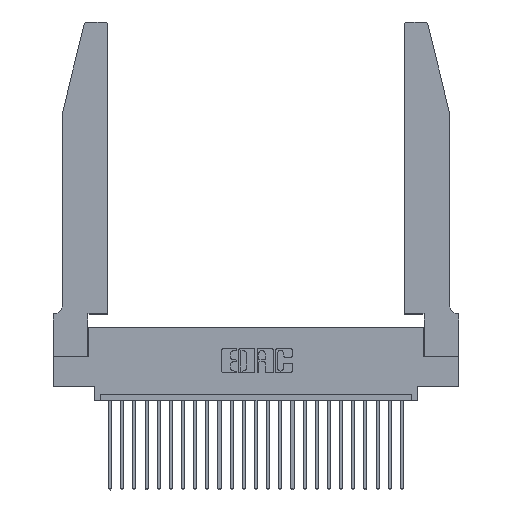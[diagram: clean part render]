
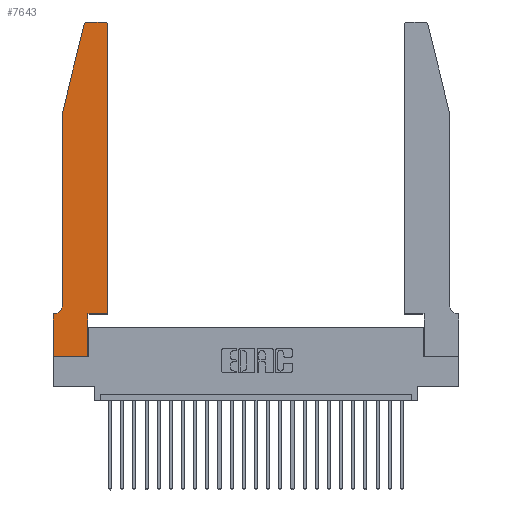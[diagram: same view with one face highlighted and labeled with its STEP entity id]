
A CAD part, top view. The second image highlights one B-rep face of the part: STEP entity #7643.
In plain terms, the highlighted planar face has unit normal (0, 0, 1).
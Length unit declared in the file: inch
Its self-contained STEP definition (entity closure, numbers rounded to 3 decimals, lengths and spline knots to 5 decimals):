
#42 = EDGE_CURVE ( 'NONE', #4178, #14159, #10183, .T. ) ;
#282 = VECTOR ( 'NONE', #21362, 39.37008 ) ;
#537 = DIRECTION ( 'NONE',  ( 1., 0., 0. ) ) ;
#866 = AXIS2_PLACEMENT_3D ( 'NONE', #18104, #2823, #10908 ) ;
#1161 = EDGE_LOOP ( 'NONE', ( #21668, #25241, #9745, #19186, #22105, #18938, #23691, #1825, #6431, #4393, #26007, #18659 ) ) ;
#1350 = CIRCLE ( 'NONE', #866, 0.07 ) ;
#1559 = LINE ( 'NONE', #8080, #11611 ) ;
#1583 = CARTESIAN_POINT ( 'NONE',  ( 0., 0.35, 0.37 ) ) ;
#1825 = ORIENTED_EDGE ( 'NONE', *, *, #9039, .T. ) ;
#1847 = EDGE_CURVE ( 'NONE', #8274, #24404, #5391, .T. ) ;
#2293 = DIRECTION ( 'NONE',  ( 0., 1., 0. ) ) ;
#2823 = DIRECTION ( 'NONE',  ( 0., 0., -1. ) ) ;
#2844 = VECTOR ( 'NONE', #20369, 39.37008 ) ;
#3102 = CARTESIAN_POINT ( 'NONE',  ( 0.0755, 2., 0.37 ) ) ;
#3602 = EDGE_CURVE ( 'NONE', #6146, #17665, #1559, .T. ) ;
#3891 = CARTESIAN_POINT ( 'NONE',  ( 0.2605, 2.75, 0.37 ) ) ;
#4178 = VERTEX_POINT ( 'NONE', #21834 ) ;
#4284 = VERTEX_POINT ( 'NONE', #10160 ) ;
#4393 = ORIENTED_EDGE ( 'NONE', *, *, #17517, .T. ) ;
#4582 = VECTOR ( 'NONE', #25202, 39.37008 ) ;
#4914 = EDGE_CURVE ( 'NONE', #7433, #5770, #16569, .T. ) ;
#5391 = LINE ( 'NONE', #12675, #2844 ) ;
#5650 = DIRECTION ( 'NONE',  ( 0., -1., 0. ) ) ;
#5770 = VERTEX_POINT ( 'NONE', #8282 ) ;
#5902 = CARTESIAN_POINT ( 'NONE',  ( 0.4205, 2.75, 0.37 ) ) ;
#6146 = VERTEX_POINT ( 'NONE', #6194 ) ;
#6194 = CARTESIAN_POINT ( 'NONE',  ( 0., 0.35, 0.37 ) ) ;
#6374 = FACE_OUTER_BOUND ( 'NONE', #1161, .T. ) ;
#6431 = ORIENTED_EDGE ( 'NONE', *, *, #18869, .T. ) ;
#6601 = CARTESIAN_POINT ( 'NONE',  ( 0.2865, 0.35, 0.37 ) ) ;
#6682 = LINE ( 'NONE', #3891, #6994 ) ;
#6994 = VECTOR ( 'NONE', #24303, 39.37008 ) ;
#7001 = EDGE_CURVE ( 'NONE', #5770, #8465, #1350, .T. ) ;
#7410 = CARTESIAN_POINT ( 'NONE',  ( 0.25487, 2.72718, 0.37 ) ) ;
#7433 = VERTEX_POINT ( 'NONE', #19551 ) ;
#7643 = ADVANCED_FACE ( 'NONE', ( #6374 ), #21573, .T. ) ;
#7696 = DIRECTION ( 'NONE',  ( 1., 0., 0. ) ) ;
#8080 = CARTESIAN_POINT ( 'NONE',  ( 0., 0., 0.37 ) ) ;
#8274 = VERTEX_POINT ( 'NONE', #15698 ) ;
#8282 = CARTESIAN_POINT ( 'NONE',  ( 0.0755, 0.42, 0.37 ) ) ;
#8408 = LINE ( 'NONE', #3102, #25663 ) ;
#8465 = VERTEX_POINT ( 'NONE', #17090 ) ;
#9039 = EDGE_CURVE ( 'NONE', #17665, #4284, #26032, .T. ) ;
#9628 = VECTOR ( 'NONE', #2293, 39.37008 ) ;
#9745 = ORIENTED_EDGE ( 'NONE', *, *, #18416, .T. ) ;
#9931 = CARTESIAN_POINT ( 'NONE',  ( 0.0755, 2., 0.37 ) ) ;
#10160 = CARTESIAN_POINT ( 'NONE',  ( 0.2865, 0., 0.37 ) ) ;
#10183 = CIRCLE ( 'NONE', #14211, 0.03 ) ;
#10206 = CIRCLE ( 'NONE', #21078, 0.03 ) ;
#10581 = VERTEX_POINT ( 'NONE', #24111 ) ;
#10833 = LINE ( 'NONE', #19227, #4582 ) ;
#10908 = DIRECTION ( 'NONE',  ( -1., 0., 0. ) ) ;
#11016 = VERTEX_POINT ( 'NONE', #5902 ) ;
#11131 = CARTESIAN_POINT ( 'NONE',  ( 0.4205, 2.72, 0.37 ) ) ;
#11213 = LINE ( 'NONE', #6601, #9628 ) ;
#11611 = VECTOR ( 'NONE', #15700, 39.37008 ) ;
#12675 = CARTESIAN_POINT ( 'NONE',  ( 0.4505, 0.35, 0.37 ) ) ;
#13285 = CARTESIAN_POINT ( 'NONE',  ( 0.4505, 0.35, 0.37 ) ) ;
#13693 = CARTESIAN_POINT ( 'NONE',  ( 0.284, 2.72, 0.37 ) ) ;
#13778 = DIRECTION ( 'NONE',  ( 0., 0., 1. ) ) ;
#14159 = VERTEX_POINT ( 'NONE', #7410 ) ;
#14211 = AXIS2_PLACEMENT_3D ( 'NONE', #13693, #13778, #17656 ) ;
#15086 = DIRECTION ( 'NONE',  ( 0., 0., 1. ) ) ;
#15698 = CARTESIAN_POINT ( 'NONE',  ( 0.4505, 0.35, 0.37 ) ) ;
#15700 = DIRECTION ( 'NONE',  ( 0., -1., 0. ) ) ;
#15930 = EDGE_CURVE ( 'NONE', #11016, #4178, #6682, .T. ) ;
#16569 = LINE ( 'NONE', #9931, #20604 ) ;
#16924 = DIRECTION ( 'NONE',  ( 1., 0., 0. ) ) ;
#17090 = CARTESIAN_POINT ( 'NONE',  ( 0.0055, 0.35, 0.37 ) ) ;
#17148 = DIRECTION ( 'NONE',  ( -0.239, -0.971, 0. ) ) ;
#17517 = EDGE_CURVE ( 'NONE', #10581, #8274, #21627, .T. ) ;
#17656 = DIRECTION ( 'NONE',  ( 1., 0., 0. ) ) ;
#17665 = VERTEX_POINT ( 'NONE', #17762 ) ;
#17762 = CARTESIAN_POINT ( 'NONE',  ( 0., 0., 0.37 ) ) ;
#18104 = CARTESIAN_POINT ( 'NONE',  ( 0.0055, 0.42, 0.37 ) ) ;
#18416 = EDGE_CURVE ( 'NONE', #14159, #7433, #8408, .T. ) ;
#18659 = ORIENTED_EDGE ( 'NONE', *, *, #20588, .T. ) ;
#18869 = EDGE_CURVE ( 'NONE', #4284, #10581, #11213, .T. ) ;
#18938 = ORIENTED_EDGE ( 'NONE', *, *, #20067, .T. ) ;
#19186 = ORIENTED_EDGE ( 'NONE', *, *, #4914, .T. ) ;
#19227 = CARTESIAN_POINT ( 'NONE',  ( 0.0755, 0.35, 0.37 ) ) ;
#19551 = CARTESIAN_POINT ( 'NONE',  ( 0.0755, 2., 0.37 ) ) ;
#20067 = EDGE_CURVE ( 'NONE', #8465, #6146, #10833, .T. ) ;
#20369 = DIRECTION ( 'NONE',  ( 0., 1., 0. ) ) ;
#20588 = EDGE_CURVE ( 'NONE', #24404, #11016, #10206, .T. ) ;
#20604 = VECTOR ( 'NONE', #5650, 39.37008 ) ;
#20675 = VECTOR ( 'NONE', #537, 39.37008 ) ;
#21078 = AXIS2_PLACEMENT_3D ( 'NONE', #11131, #15086, #16924 ) ;
#21362 = DIRECTION ( 'NONE',  ( 1., 0., 0. ) ) ;
#21368 = CARTESIAN_POINT ( 'NONE',  ( 0.4505, 2.72, 0.37 ) ) ;
#21573 = PLANE ( 'NONE',  #25935 ) ;
#21627 = LINE ( 'NONE', #13285, #282 ) ;
#21668 = ORIENTED_EDGE ( 'NONE', *, *, #15930, .T. ) ;
#21834 = CARTESIAN_POINT ( 'NONE',  ( 0.284, 2.75, 0.37 ) ) ;
#22105 = ORIENTED_EDGE ( 'NONE', *, *, #7001, .T. ) ;
#23691 = ORIENTED_EDGE ( 'NONE', *, *, #3602, .T. ) ;
#23873 = CARTESIAN_POINT ( 'NONE',  ( 0., 0., 0.37 ) ) ;
#24111 = CARTESIAN_POINT ( 'NONE',  ( 0.2865, 0.35, 0.37 ) ) ;
#24303 = DIRECTION ( 'NONE',  ( -1., 0., 0. ) ) ;
#24404 = VERTEX_POINT ( 'NONE', #21368 ) ;
#25202 = DIRECTION ( 'NONE',  ( -1., 0., 0. ) ) ;
#25241 = ORIENTED_EDGE ( 'NONE', *, *, #42, .T. ) ;
#25557 = DIRECTION ( 'NONE',  ( 0., 0., 1. ) ) ;
#25663 = VECTOR ( 'NONE', #17148, 39.37008 ) ;
#25935 = AXIS2_PLACEMENT_3D ( 'NONE', #1583, #25557, #7696 ) ;
#26007 = ORIENTED_EDGE ( 'NONE', *, *, #1847, .T. ) ;
#26032 = LINE ( 'NONE', #23873, #20675 ) ;
